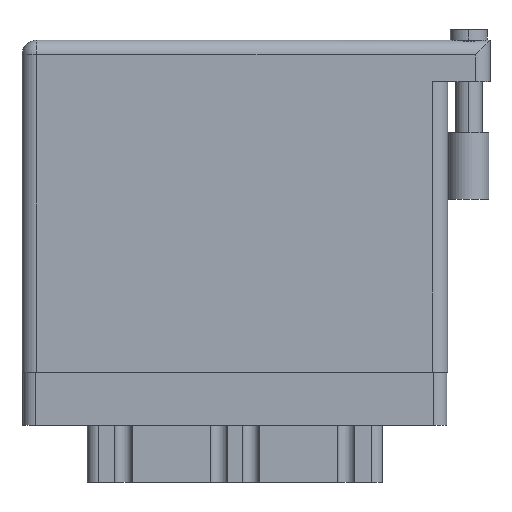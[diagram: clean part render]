
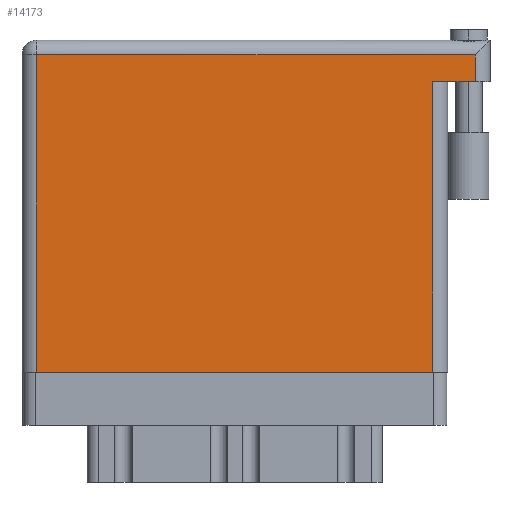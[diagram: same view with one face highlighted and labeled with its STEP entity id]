
A CAD part, front view. The second image highlights one B-rep face of the part: STEP entity #14173.
In plain terms, the highlighted face is planar.
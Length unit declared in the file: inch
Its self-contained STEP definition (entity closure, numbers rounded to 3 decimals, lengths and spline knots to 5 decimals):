
#787 = CARTESIAN_POINT ( 'NONE',  ( 1.938, 0., 0. ) ) ;
#3352 = VECTOR ( 'NONE', #17353, 39.37008 ) ;
#3805 = CARTESIAN_POINT ( 'NONE',  ( 0.07, 0., 0. ) ) ;
#4455 = VECTOR ( 'NONE', #19249, 39.37008 ) ;
#4794 = VECTOR ( 'NONE', #24681, 39.37008 ) ;
#4891 = VERTEX_POINT ( 'NONE', #10673 ) ;
#5602 = LINE ( 'NONE', #19487, #33249 ) ;
#5883 = CARTESIAN_POINT ( 'NONE',  ( 2.208, 1.369, 0. ) ) ;
#6028 = ORIENTED_EDGE ( 'NONE', *, *, #10522, .T. ) ;
#6771 = CARTESIAN_POINT ( 'NONE',  ( 0., 0., 0. ) ) ;
#6949 = VERTEX_POINT ( 'NONE', #9066 ) ;
#7167 = ORIENTED_EDGE ( 'NONE', *, *, #29132, .T. ) ;
#7617 = CARTESIAN_POINT ( 'NONE',  ( 1.938, 1.369, 0. ) ) ;
#7833 = EDGE_LOOP ( 'NONE', ( #13044, #26306, #10683, #7167, #19170, #6028 ) ) ;
#8660 = LINE ( 'NONE', #5883, #4455 ) ;
#8866 = LINE ( 'NONE', #6771, #3352 ) ;
#9066 = CARTESIAN_POINT ( 'NONE',  ( 0.07, 1.496, 0. ) ) ;
#10522 = EDGE_CURVE ( 'NONE', #6949, #28753, #27276, .T. ) ;
#10673 = CARTESIAN_POINT ( 'NONE',  ( 2.138, 1.369, 0. ) ) ;
#10683 = ORIENTED_EDGE ( 'NONE', *, *, #22221, .F. ) ;
#12948 = CARTESIAN_POINT ( 'NONE',  ( 0., 1.496, 0. ) ) ;
#13044 = ORIENTED_EDGE ( 'NONE', *, *, #23716, .T. ) ;
#13323 = LINE ( 'NONE', #7617, #22805 ) ;
#14080 = DIRECTION ( 'NONE',  ( 0., 1., 0. ) ) ;
#14173 = ADVANCED_FACE ( 'NONE', ( #15119 ), #15642, .F. ) ;
#15119 = FACE_OUTER_BOUND ( 'NONE', #7833, .T. ) ;
#15642 = PLANE ( 'NONE',  #27349 ) ;
#16983 = CARTESIAN_POINT ( 'NONE',  ( 2.138, 1.496, 0. ) ) ;
#17353 = DIRECTION ( 'NONE',  ( 1., 0., 0. ) ) ;
#17910 = CARTESIAN_POINT ( 'NONE',  ( 0., 1.566, 0. ) ) ;
#19170 = ORIENTED_EDGE ( 'NONE', *, *, #32735, .T. ) ;
#19249 = DIRECTION ( 'NONE',  ( -1., 0., 0. ) ) ;
#19487 = CARTESIAN_POINT ( 'NONE',  ( 2.138, 1.566, 0. ) ) ;
#20266 = VERTEX_POINT ( 'NONE', #16983 ) ;
#20655 = VERTEX_POINT ( 'NONE', #787 ) ;
#22221 = EDGE_CURVE ( 'NONE', #4891, #34271, #8660, .T. ) ;
#22805 = VECTOR ( 'NONE', #23775, 39.37008 ) ;
#23219 = LINE ( 'NONE', #12948, #30604 ) ;
#23314 = DIRECTION ( 'NONE',  ( 0., 0., -1. ) ) ;
#23716 = EDGE_CURVE ( 'NONE', #28753, #20655, #8866, .T. ) ;
#23775 = DIRECTION ( 'NONE',  ( 0., 1., 0. ) ) ;
#24681 = DIRECTION ( 'NONE',  ( 0., -1., 0. ) ) ;
#26047 = CARTESIAN_POINT ( 'NONE',  ( 1.938, 1.369, 0. ) ) ;
#26306 = ORIENTED_EDGE ( 'NONE', *, *, #32314, .T. ) ;
#27276 = LINE ( 'NONE', #3805, #4794 ) ;
#27349 = AXIS2_PLACEMENT_3D ( 'NONE', #17910, #23314, #33906 ) ;
#28753 = VERTEX_POINT ( 'NONE', #31129 ) ;
#29113 = DIRECTION ( 'NONE',  ( -1., 0., 0. ) ) ;
#29132 = EDGE_CURVE ( 'NONE', #4891, #20266, #5602, .T. ) ;
#30604 = VECTOR ( 'NONE', #29113, 39.37008 ) ;
#31129 = CARTESIAN_POINT ( 'NONE',  ( 0.07, 0., 0. ) ) ;
#32314 = EDGE_CURVE ( 'NONE', #20655, #34271, #13323, .T. ) ;
#32735 = EDGE_CURVE ( 'NONE', #20266, #6949, #23219, .T. ) ;
#33249 = VECTOR ( 'NONE', #14080, 39.37008 ) ;
#33906 = DIRECTION ( 'NONE',  ( -1., 0., 0. ) ) ;
#34271 = VERTEX_POINT ( 'NONE', #26047 ) ;
